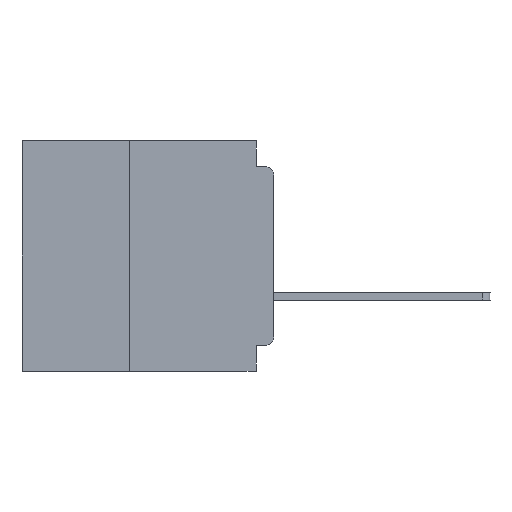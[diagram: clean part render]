
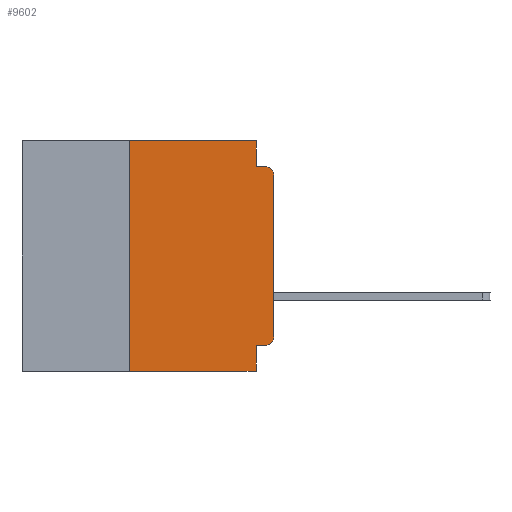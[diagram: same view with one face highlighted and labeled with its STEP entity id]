
A CAD part, left-side view. The second image highlights one B-rep face of the part: STEP entity #9602.
In plain terms, the highlighted planar face has unit normal (-1, 0, 0).
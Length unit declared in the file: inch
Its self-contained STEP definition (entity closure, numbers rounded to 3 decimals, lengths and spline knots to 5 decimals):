
#432 = VERTEX_POINT ( 'NONE', #53173 ) ;
#894 = DIRECTION ( 'NONE',  ( 0., 1., 0. ) ) ;
#1045 = CARTESIAN_POINT ( 'NONE',  ( 0., 0.031, -0.355 ) ) ;
#1917 = LINE ( 'NONE', #53150, #12361 ) ;
#2022 = DIRECTION ( 'NONE',  ( 0., 0., 1. ) ) ;
#3825 = DIRECTION ( 'NONE',  ( 0., -1., 0. ) ) ;
#4126 = LINE ( 'NONE', #18606, #55816 ) ;
#5386 = DIRECTION ( 'NONE',  ( -1., 0., 0. ) ) ;
#5762 = ORIENTED_EDGE ( 'NONE', *, *, #46307, .F. ) ;
#6320 = CARTESIAN_POINT ( 'NONE',  ( 0., 0., 0. ) ) ;
#6623 = VERTEX_POINT ( 'NONE', #9715 ) ;
#6736 = CARTESIAN_POINT ( 'NONE',  ( 0., 0.015, -0.355 ) ) ;
#6790 = CARTESIAN_POINT ( 'NONE',  ( 0., 0.031, -0.4 ) ) ;
#7347 = EDGE_CURVE ( 'NONE', #6623, #432, #37047, .T. ) ;
#7379 = VECTOR ( 'NONE', #33289, 39.37008 ) ;
#8047 = ORIENTED_EDGE ( 'NONE', *, *, #32748, .F. ) ;
#8083 = DIRECTION ( 'NONE',  ( 0., -1., 0. ) ) ;
#9255 = DIRECTION ( 'NONE',  ( 0., -1., 0. ) ) ;
#9278 = DIRECTION ( 'NONE',  ( -1., 0., 0. ) ) ;
#9602 = ADVANCED_FACE ( 'NONE', ( #21704 ), #33011, .F. ) ;
#9715 = CARTESIAN_POINT ( 'NONE',  ( 0., 0.031, 0. ) ) ;
#10913 = EDGE_CURVE ( 'NONE', #432, #15960, #42163, .T. ) ;
#10927 = CARTESIAN_POINT ( 'NONE',  ( 0., 0., -0.06 ) ) ;
#10980 = DIRECTION ( 'NONE',  ( 0., 0., -1. ) ) ;
#12361 = VECTOR ( 'NONE', #9255, 39.37008 ) ;
#13563 = VECTOR ( 'NONE', #17282, 39.37008 ) ;
#13649 = VERTEX_POINT ( 'NONE', #42815 ) ;
#14367 = AXIS2_PLACEMENT_3D ( 'NONE', #32817, #37443, #10980 ) ;
#15451 = CIRCLE ( 'NONE', #33258, 0.015 ) ;
#15776 = ORIENTED_EDGE ( 'NONE', *, *, #7347, .F. ) ;
#15960 = VERTEX_POINT ( 'NONE', #39388 ) ;
#16064 = EDGE_CURVE ( 'NONE', #53730, #13649, #1917, .T. ) ;
#17282 = DIRECTION ( 'NONE',  ( 0., 0., -1. ) ) ;
#18606 = CARTESIAN_POINT ( 'NONE',  ( 0., 0., -0.355 ) ) ;
#19499 = EDGE_CURVE ( 'NONE', #50545, #13649, #42608, .T. ) ;
#20043 = CARTESIAN_POINT ( 'NONE',  ( 0., 0.25, 0. ) ) ;
#21704 = FACE_OUTER_BOUND ( 'NONE', #29243, .T. ) ;
#25701 = CARTESIAN_POINT ( 'NONE',  ( 0., 0., -0.045 ) ) ;
#27647 = CARTESIAN_POINT ( 'NONE',  ( 0., 0.25, -0.4 ) ) ;
#28620 = EDGE_CURVE ( 'NONE', #31077, #15960, #51598, .T. ) ;
#29243 = EDGE_LOOP ( 'NONE', ( #53025, #48925, #45034, #15776, #8047, #5762, #55978, #34547, #47727, #50741 ) ) ;
#30460 = VECTOR ( 'NONE', #8083, 39.37008 ) ;
#31077 = VERTEX_POINT ( 'NONE', #10927 ) ;
#31909 = CARTESIAN_POINT ( 'NONE',  ( 0., 0.015, -0.34 ) ) ;
#32491 = LINE ( 'NONE', #52263, #54434 ) ;
#32748 = EDGE_CURVE ( 'NONE', #54478, #6623, #32491, .T. ) ;
#32817 = CARTESIAN_POINT ( 'NONE',  ( 0., 0.437, 0. ) ) ;
#33011 = PLANE ( 'NONE',  #14367 ) ;
#33258 = AXIS2_PLACEMENT_3D ( 'NONE', #31909, #5386, #36371 ) ;
#33289 = DIRECTION ( 'NONE',  ( 0., 0., -1. ) ) ;
#33539 = VECTOR ( 'NONE', #55004, 39.37008 ) ;
#34547 = ORIENTED_EDGE ( 'NONE', *, *, #19499, .F. ) ;
#35770 = CARTESIAN_POINT ( 'NONE',  ( 0., 0.015, -0.06 ) ) ;
#36323 = LINE ( 'NONE', #50656, #33539 ) ;
#36371 = DIRECTION ( 'NONE',  ( 0., 0., -1. ) ) ;
#37047 = LINE ( 'NONE', #43637, #13563 ) ;
#37443 = DIRECTION ( 'NONE',  ( 1., 0., 0. ) ) ;
#37578 = CARTESIAN_POINT ( 'NONE',  ( 0., 0., -0.34 ) ) ;
#37741 = EDGE_CURVE ( 'NONE', #51934, #50545, #4126, .T. ) ;
#39388 = CARTESIAN_POINT ( 'NONE',  ( 0., 0.015, -0.045 ) ) ;
#40183 = DIRECTION ( 'NONE',  ( 0., 0., -1. ) ) ;
#40298 = EDGE_CURVE ( 'NONE', #52736, #31077, #44698, .T. ) ;
#42163 = LINE ( 'NONE', #25701, #30460 ) ;
#42208 = EDGE_CURVE ( 'NONE', #51934, #52736, #15451, .T. ) ;
#42608 = LINE ( 'NONE', #6790, #7379 ) ;
#42815 = CARTESIAN_POINT ( 'NONE',  ( 0., 0.031, -0.4 ) ) ;
#43637 = CARTESIAN_POINT ( 'NONE',  ( 0., 0.031, 0. ) ) ;
#44698 = LINE ( 'NONE', #6320, #54911 ) ;
#45034 = ORIENTED_EDGE ( 'NONE', *, *, #10913, .F. ) ;
#46307 = EDGE_CURVE ( 'NONE', #53730, #54478, #36323, .T. ) ;
#47727 = ORIENTED_EDGE ( 'NONE', *, *, #37741, .F. ) ;
#48925 = ORIENTED_EDGE ( 'NONE', *, *, #28620, .T. ) ;
#49006 = AXIS2_PLACEMENT_3D ( 'NONE', #35770, #9278, #40183 ) ;
#50545 = VERTEX_POINT ( 'NONE', #1045 ) ;
#50656 = CARTESIAN_POINT ( 'NONE',  ( 0., 0.25, -0.4 ) ) ;
#50741 = ORIENTED_EDGE ( 'NONE', *, *, #42208, .T. ) ;
#51598 = CIRCLE ( 'NONE', #49006, 0.015 ) ;
#51934 = VERTEX_POINT ( 'NONE', #6736 ) ;
#52263 = CARTESIAN_POINT ( 'NONE',  ( 0., 0.437, 0. ) ) ;
#52736 = VERTEX_POINT ( 'NONE', #37578 ) ;
#53025 = ORIENTED_EDGE ( 'NONE', *, *, #40298, .T. ) ;
#53150 = CARTESIAN_POINT ( 'NONE',  ( 0., 0.437, -0.4 ) ) ;
#53173 = CARTESIAN_POINT ( 'NONE',  ( 0., 0.031, -0.045 ) ) ;
#53730 = VERTEX_POINT ( 'NONE', #27647 ) ;
#54434 = VECTOR ( 'NONE', #3825, 39.37008 ) ;
#54478 = VERTEX_POINT ( 'NONE', #20043 ) ;
#54911 = VECTOR ( 'NONE', #2022, 39.37008 ) ;
#55004 = DIRECTION ( 'NONE',  ( 0., 0., 1. ) ) ;
#55816 = VECTOR ( 'NONE', #894, 39.37008 ) ;
#55978 = ORIENTED_EDGE ( 'NONE', *, *, #16064, .T. ) ;
